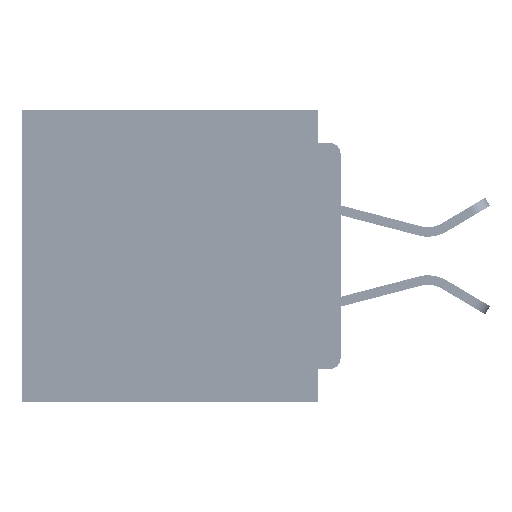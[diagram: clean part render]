
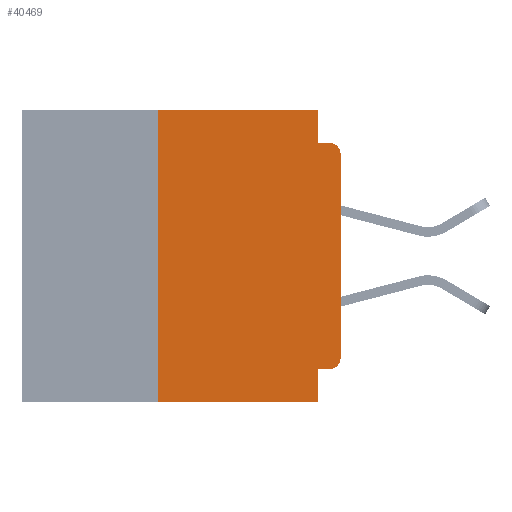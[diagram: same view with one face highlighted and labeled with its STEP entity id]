
A CAD part, left-side view. The second image highlights one B-rep face of the part: STEP entity #40469.
In plain terms, the highlighted planar face has unit normal (-1, 0, 0).
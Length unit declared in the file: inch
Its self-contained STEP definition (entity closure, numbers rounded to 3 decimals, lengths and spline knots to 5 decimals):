
#585 = ORIENTED_EDGE ( 'NONE', *, *, #28061, .F. ) ;
#1248 = DIRECTION ( 'NONE',  ( 0., -1., 0. ) ) ;
#1784 = DIRECTION ( 'NONE',  ( 0., -1., 0. ) ) ;
#4044 = AXIS2_PLACEMENT_3D ( 'NONE', #36275, #11634, #40421 ) ;
#4465 = LINE ( 'NONE', #9465, #49672 ) ;
#4582 = ORIENTED_EDGE ( 'NONE', *, *, #50130, .F. ) ;
#4674 = DIRECTION ( 'NONE',  ( 0., 0., 1. ) ) ;
#5846 = CARTESIAN_POINT ( 'NONE',  ( 0., 0.031, -0.4 ) ) ;
#6633 = ORIENTED_EDGE ( 'NONE', *, *, #38355, .T. ) ;
#7279 = VERTEX_POINT ( 'NONE', #52792 ) ;
#7675 = VERTEX_POINT ( 'NONE', #5846 ) ;
#8151 = LINE ( 'NONE', #53323, #28833 ) ;
#8924 = LINE ( 'NONE', #22425, #28312 ) ;
#9057 = CARTESIAN_POINT ( 'NONE',  ( 0., 0., -0.355 ) ) ;
#9465 = CARTESIAN_POINT ( 'NONE',  ( 0., 0.437, -0.4 ) ) ;
#9524 = CARTESIAN_POINT ( 'NONE',  ( 0., 0.015, -0.34 ) ) ;
#9869 = CARTESIAN_POINT ( 'NONE',  ( 0., 0.031, -0.355 ) ) ;
#10744 = EDGE_CURVE ( 'NONE', #31727, #7279, #8151, .T. ) ;
#11034 = VERTEX_POINT ( 'NONE', #9869 ) ;
#11110 = CARTESIAN_POINT ( 'NONE',  ( 0., 0.031, -0.4 ) ) ;
#11222 = EDGE_CURVE ( 'NONE', #11034, #7675, #39711, .T. ) ;
#11634 = DIRECTION ( 'NONE',  ( 1., 0., 0. ) ) ;
#12009 = EDGE_CURVE ( 'NONE', #40143, #26608, #24163, .T. ) ;
#13684 = DIRECTION ( 'NONE',  ( 0., 0., -1. ) ) ;
#13949 = AXIS2_PLACEMENT_3D ( 'NONE', #19538, #48370, #23681 ) ;
#14008 = CIRCLE ( 'NONE', #13949, 0.015 ) ;
#14475 = ORIENTED_EDGE ( 'NONE', *, *, #11222, .F. ) ;
#15274 = EDGE_LOOP ( 'NONE', ( #53328, #46787, #32222, #23227, #585, #41554, #6633, #14475, #4582, #42915 ) ) ;
#16802 = VECTOR ( 'NONE', #48302, 39.37008 ) ;
#17277 = VERTEX_POINT ( 'NONE', #18751 ) ;
#18586 = DIRECTION ( 'NONE',  ( 0., -1., 0. ) ) ;
#18751 = CARTESIAN_POINT ( 'NONE',  ( 0., 0.015, -0.355 ) ) ;
#19538 = CARTESIAN_POINT ( 'NONE',  ( 0., 0.015, -0.06 ) ) ;
#20570 = LINE ( 'NONE', #22713, #41195 ) ;
#22425 = CARTESIAN_POINT ( 'NONE',  ( 0., 0., -0.045 ) ) ;
#22713 = CARTESIAN_POINT ( 'NONE',  ( 0., 0.437, 0. ) ) ;
#23227 = ORIENTED_EDGE ( 'NONE', *, *, #48131, .F. ) ;
#23377 = CARTESIAN_POINT ( 'NONE',  ( 0., 0.015, -0.045 ) ) ;
#23681 = DIRECTION ( 'NONE',  ( 0., 0., -1. ) ) ;
#24163 = LINE ( 'NONE', #33562, #46062 ) ;
#25479 = DIRECTION ( 'NONE',  ( 0., 1., 0. ) ) ;
#26608 = VERTEX_POINT ( 'NONE', #45313 ) ;
#26796 = VERTEX_POINT ( 'NONE', #50793 ) ;
#27536 = DIRECTION ( 'NONE',  ( 0., 0., -1. ) ) ;
#27802 = CARTESIAN_POINT ( 'NONE',  ( 0., 0.031, 0. ) ) ;
#28061 = EDGE_CURVE ( 'NONE', #26608, #26796, #20570, .T. ) ;
#28312 = VECTOR ( 'NONE', #1784, 39.37008 ) ;
#28833 = VECTOR ( 'NONE', #49188, 39.37008 ) ;
#31727 = VERTEX_POINT ( 'NONE', #50495 ) ;
#32222 = ORIENTED_EDGE ( 'NONE', *, *, #49208, .F. ) ;
#33562 = CARTESIAN_POINT ( 'NONE',  ( 0., 0.25, -0.4 ) ) ;
#35334 = CARTESIAN_POINT ( 'NONE',  ( 0., 0.031, -0.045 ) ) ;
#36275 = CARTESIAN_POINT ( 'NONE',  ( 0., 0.437, 0. ) ) ;
#37151 = EDGE_CURVE ( 'NONE', #17277, #31727, #42034, .T. ) ;
#37562 = CARTESIAN_POINT ( 'NONE',  ( 0., 0.25, -0.4 ) ) ;
#37821 = VECTOR ( 'NONE', #25479, 39.37008 ) ;
#38338 = DIRECTION ( 'NONE',  ( -1., 0., 0. ) ) ;
#38355 = EDGE_CURVE ( 'NONE', #40143, #7675, #4465, .T. ) ;
#39711 = LINE ( 'NONE', #11110, #49411 ) ;
#40143 = VERTEX_POINT ( 'NONE', #37562 ) ;
#40421 = DIRECTION ( 'NONE',  ( 0., 0., -1. ) ) ;
#40469 = ADVANCED_FACE ( 'NONE', ( #50155 ), #52707, .F. ) ;
#41195 = VECTOR ( 'NONE', #18586, 39.37008 ) ;
#41554 = ORIENTED_EDGE ( 'NONE', *, *, #12009, .F. ) ;
#42034 = CIRCLE ( 'NONE', #46783, 0.015 ) ;
#42915 = ORIENTED_EDGE ( 'NONE', *, *, #37151, .T. ) ;
#44852 = VERTEX_POINT ( 'NONE', #35334 ) ;
#45313 = CARTESIAN_POINT ( 'NONE',  ( 0., 0.25, 0. ) ) ;
#46062 = VECTOR ( 'NONE', #4674, 39.37008 ) ;
#46231 = EDGE_CURVE ( 'NONE', #7279, #48762, #14008, .T. ) ;
#46783 = AXIS2_PLACEMENT_3D ( 'NONE', #9524, #38338, #13684 ) ;
#46787 = ORIENTED_EDGE ( 'NONE', *, *, #46231, .T. ) ;
#48131 = EDGE_CURVE ( 'NONE', #26796, #44852, #49706, .T. ) ;
#48302 = DIRECTION ( 'NONE',  ( 0., 0., -1. ) ) ;
#48370 = DIRECTION ( 'NONE',  ( -1., 0., 0. ) ) ;
#48762 = VERTEX_POINT ( 'NONE', #23377 ) ;
#48811 = LINE ( 'NONE', #9057, #37821 ) ;
#49188 = DIRECTION ( 'NONE',  ( 0., 0., 1. ) ) ;
#49208 = EDGE_CURVE ( 'NONE', #44852, #48762, #8924, .T. ) ;
#49411 = VECTOR ( 'NONE', #27536, 39.37008 ) ;
#49672 = VECTOR ( 'NONE', #1248, 39.37008 ) ;
#49706 = LINE ( 'NONE', #27802, #16802 ) ;
#50130 = EDGE_CURVE ( 'NONE', #17277, #11034, #48811, .T. ) ;
#50155 = FACE_OUTER_BOUND ( 'NONE', #15274, .T. ) ;
#50495 = CARTESIAN_POINT ( 'NONE',  ( 0., 0., -0.34 ) ) ;
#50793 = CARTESIAN_POINT ( 'NONE',  ( 0., 0.031, 0. ) ) ;
#52707 = PLANE ( 'NONE',  #4044 ) ;
#52792 = CARTESIAN_POINT ( 'NONE',  ( 0., 0., -0.06 ) ) ;
#53323 = CARTESIAN_POINT ( 'NONE',  ( 0., 0., 0. ) ) ;
#53328 = ORIENTED_EDGE ( 'NONE', *, *, #10744, .T. ) ;
